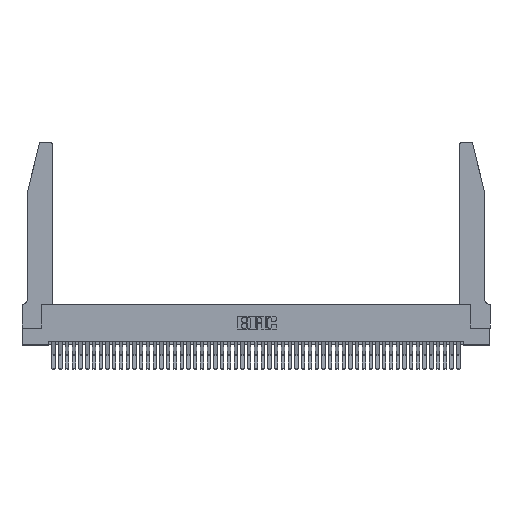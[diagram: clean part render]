
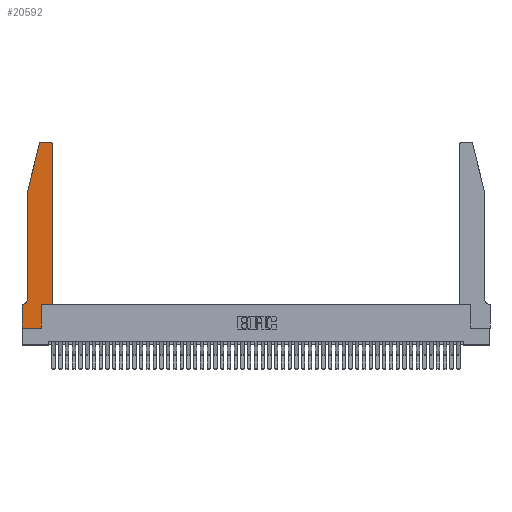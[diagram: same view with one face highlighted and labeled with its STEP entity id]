
A CAD part, top view. The second image highlights one B-rep face of the part: STEP entity #20592.
In plain terms, the highlighted planar face has unit normal (0, 0, 1).
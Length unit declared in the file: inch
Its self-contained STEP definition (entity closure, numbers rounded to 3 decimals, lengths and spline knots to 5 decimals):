
#736 = CARTESIAN_POINT ( 'NONE',  ( 0.2865, 0.35, 0.37 ) ) ;
#849 = VERTEX_POINT ( 'NONE', #40223 ) ;
#1728 = EDGE_CURVE ( 'NONE', #849, #7558, #12111, .T. ) ;
#2448 = DIRECTION ( 'NONE',  ( 0., 0., 1. ) ) ;
#2613 = PLANE ( 'NONE',  #36072 ) ;
#3341 = VECTOR ( 'NONE', #44557, 39.37008 ) ;
#3470 = CIRCLE ( 'NONE', #30653, 0.07 ) ;
#4839 = CARTESIAN_POINT ( 'NONE',  ( 0.0055, 0.42, 0.37 ) ) ;
#5126 = VECTOR ( 'NONE', #8208, 39.37008 ) ;
#5716 = LINE ( 'NONE', #25423, #48754 ) ;
#6381 = DIRECTION ( 'NONE',  ( 0., 0., 1. ) ) ;
#6722 = EDGE_CURVE ( 'NONE', #35394, #10743, #24984, .T. ) ;
#6823 = CARTESIAN_POINT ( 'NONE',  ( 0.0755, 0.42, 0.37 ) ) ;
#7558 = VERTEX_POINT ( 'NONE', #49541 ) ;
#8086 = DIRECTION ( 'NONE',  ( 1., 0., 0. ) ) ;
#8208 = DIRECTION ( 'NONE',  ( -1., 0., 0. ) ) ;
#8574 = EDGE_CURVE ( 'NONE', #33570, #36423, #24547, .T. ) ;
#8963 = ORIENTED_EDGE ( 'NONE', *, *, #20958, .T. ) ;
#10491 = LINE ( 'NONE', #19173, #17702 ) ;
#10743 = VERTEX_POINT ( 'NONE', #35698 ) ;
#11559 = ORIENTED_EDGE ( 'NONE', *, *, #17684, .T. ) ;
#12107 = EDGE_CURVE ( 'NONE', #21826, #35394, #18662, .T. ) ;
#12111 = CIRCLE ( 'NONE', #35850, 0.03 ) ;
#12743 = EDGE_CURVE ( 'NONE', #46279, #33570, #3470, .T. ) ;
#12937 = CARTESIAN_POINT ( 'NONE',  ( 0.2605, 2.75, 0.37 ) ) ;
#13333 = ORIENTED_EDGE ( 'NONE', *, *, #31233, .T. ) ;
#14572 = VERTEX_POINT ( 'NONE', #21999 ) ;
#15708 = VECTOR ( 'NONE', #30318, 39.37008 ) ;
#15732 = ORIENTED_EDGE ( 'NONE', *, *, #28621, .T. ) ;
#17684 = EDGE_CURVE ( 'NONE', #45283, #40536, #23933, .T. ) ;
#17702 = VECTOR ( 'NONE', #30272, 39.37008 ) ;
#18358 = FACE_OUTER_BOUND ( 'NONE', #43403, .T. ) ;
#18612 = DIRECTION ( 'NONE',  ( 0., 1., 0. ) ) ;
#18662 = LINE ( 'NONE', #22224, #48422 ) ;
#19173 = CARTESIAN_POINT ( 'NONE',  ( 0., 0., 0.37 ) ) ;
#19547 = CARTESIAN_POINT ( 'NONE',  ( 0.0755, 2., 0.37 ) ) ;
#20592 = ADVANCED_FACE ( 'NONE', ( #18358 ), #2613, .T. ) ;
#20610 = CARTESIAN_POINT ( 'NONE',  ( 0., 0.35, 0.37 ) ) ;
#20958 = EDGE_CURVE ( 'NONE', #10743, #849, #38297, .T. ) ;
#21826 = VERTEX_POINT ( 'NONE', #28171 ) ;
#21999 = CARTESIAN_POINT ( 'NONE',  ( 0.0755, 2., 0.37 ) ) ;
#22224 = CARTESIAN_POINT ( 'NONE',  ( 0.4505, 0.35, 0.37 ) ) ;
#22269 = DIRECTION ( 'NONE',  ( 1., 0., 0. ) ) ;
#23768 = DIRECTION ( 'NONE',  ( -1., 0., 0. ) ) ;
#23845 = DIRECTION ( 'NONE',  ( 0., 0., 1. ) ) ;
#23933 = LINE ( 'NONE', #43524, #46987 ) ;
#24547 = LINE ( 'NONE', #42294, #5126 ) ;
#24984 = CIRCLE ( 'NONE', #29845, 0.03 ) ;
#25349 = EDGE_CURVE ( 'NONE', #37192, #45283, #39739, .T. ) ;
#25387 = ORIENTED_EDGE ( 'NONE', *, *, #8574, .T. ) ;
#25423 = CARTESIAN_POINT ( 'NONE',  ( 0.4505, 0.35, 0.37 ) ) ;
#26613 = LINE ( 'NONE', #19547, #41194 ) ;
#27046 = ORIENTED_EDGE ( 'NONE', *, *, #38594, .T. ) ;
#28171 = CARTESIAN_POINT ( 'NONE',  ( 0.4505, 0.35, 0.37 ) ) ;
#28559 = DIRECTION ( 'NONE',  ( 0., 0., -1. ) ) ;
#28621 = EDGE_CURVE ( 'NONE', #7558, #14572, #26613, .T. ) ;
#29845 = AXIS2_PLACEMENT_3D ( 'NONE', #33658, #6381, #37074 ) ;
#30218 = CARTESIAN_POINT ( 'NONE',  ( 0.2865, 0., 0.37 ) ) ;
#30272 = DIRECTION ( 'NONE',  ( 0., -1., 0. ) ) ;
#30318 = DIRECTION ( 'NONE',  ( 0., -1., 0. ) ) ;
#30653 = AXIS2_PLACEMENT_3D ( 'NONE', #4839, #28559, #48044 ) ;
#31233 = EDGE_CURVE ( 'NONE', #40536, #21826, #5716, .T. ) ;
#31305 = CARTESIAN_POINT ( 'NONE',  ( 0.284, 2.72, 0.37 ) ) ;
#32648 = LINE ( 'NONE', #46061, #15708 ) ;
#32857 = VECTOR ( 'NONE', #23768, 39.37008 ) ;
#33294 = CARTESIAN_POINT ( 'NONE',  ( 0., 0.35, 0.37 ) ) ;
#33314 = ORIENTED_EDGE ( 'NONE', *, *, #25349, .T. ) ;
#33570 = VERTEX_POINT ( 'NONE', #46287 ) ;
#33658 = CARTESIAN_POINT ( 'NONE',  ( 0.4205, 2.72, 0.37 ) ) ;
#34039 = ORIENTED_EDGE ( 'NONE', *, *, #1728, .T. ) ;
#34592 = CARTESIAN_POINT ( 'NONE',  ( 0., 0., 0.37 ) ) ;
#35346 = DIRECTION ( 'NONE',  ( -0.239, -0.971, 0. ) ) ;
#35394 = VERTEX_POINT ( 'NONE', #45111 ) ;
#35698 = CARTESIAN_POINT ( 'NONE',  ( 0.4205, 2.75, 0.37 ) ) ;
#35850 = AXIS2_PLACEMENT_3D ( 'NONE', #31305, #23845, #8086 ) ;
#36072 = AXIS2_PLACEMENT_3D ( 'NONE', #33294, #2448, #22269 ) ;
#36423 = VERTEX_POINT ( 'NONE', #20610 ) ;
#37074 = DIRECTION ( 'NONE',  ( 1., 0., 0. ) ) ;
#37192 = VERTEX_POINT ( 'NONE', #34592 ) ;
#38297 = LINE ( 'NONE', #12937, #32857 ) ;
#38594 = EDGE_CURVE ( 'NONE', #36423, #37192, #10491, .T. ) ;
#39739 = LINE ( 'NONE', #48276, #3341 ) ;
#40223 = CARTESIAN_POINT ( 'NONE',  ( 0.284, 2.75, 0.37 ) ) ;
#40536 = VERTEX_POINT ( 'NONE', #736 ) ;
#40854 = DIRECTION ( 'NONE',  ( 1., 0., 0. ) ) ;
#41124 = ORIENTED_EDGE ( 'NONE', *, *, #6722, .T. ) ;
#41194 = VECTOR ( 'NONE', #35346, 39.37008 ) ;
#42294 = CARTESIAN_POINT ( 'NONE',  ( 0.0755, 0.35, 0.37 ) ) ;
#42586 = ORIENTED_EDGE ( 'NONE', *, *, #44286, .T. ) ;
#43200 = DIRECTION ( 'NONE',  ( 0., 1., 0. ) ) ;
#43403 = EDGE_LOOP ( 'NONE', ( #8963, #34039, #15732, #42586, #44042, #25387, #27046, #33314, #11559, #13333, #49401, #41124 ) ) ;
#43524 = CARTESIAN_POINT ( 'NONE',  ( 0.2865, 0.35, 0.37 ) ) ;
#44042 = ORIENTED_EDGE ( 'NONE', *, *, #12743, .T. ) ;
#44286 = EDGE_CURVE ( 'NONE', #14572, #46279, #32648, .T. ) ;
#44557 = DIRECTION ( 'NONE',  ( 1., 0., 0. ) ) ;
#45111 = CARTESIAN_POINT ( 'NONE',  ( 0.4505, 2.72, 0.37 ) ) ;
#45283 = VERTEX_POINT ( 'NONE', #30218 ) ;
#46061 = CARTESIAN_POINT ( 'NONE',  ( 0.0755, 2., 0.37 ) ) ;
#46279 = VERTEX_POINT ( 'NONE', #6823 ) ;
#46287 = CARTESIAN_POINT ( 'NONE',  ( 0.0055, 0.35, 0.37 ) ) ;
#46987 = VECTOR ( 'NONE', #43200, 39.37008 ) ;
#48044 = DIRECTION ( 'NONE',  ( -1., 0., 0. ) ) ;
#48276 = CARTESIAN_POINT ( 'NONE',  ( 0., 0., 0.37 ) ) ;
#48422 = VECTOR ( 'NONE', #18612, 39.37008 ) ;
#48754 = VECTOR ( 'NONE', #40854, 39.37008 ) ;
#49401 = ORIENTED_EDGE ( 'NONE', *, *, #12107, .T. ) ;
#49541 = CARTESIAN_POINT ( 'NONE',  ( 0.25487, 2.72718, 0.37 ) ) ;
